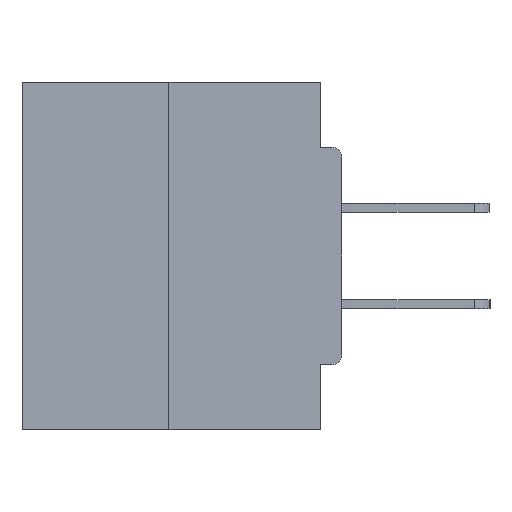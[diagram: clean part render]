
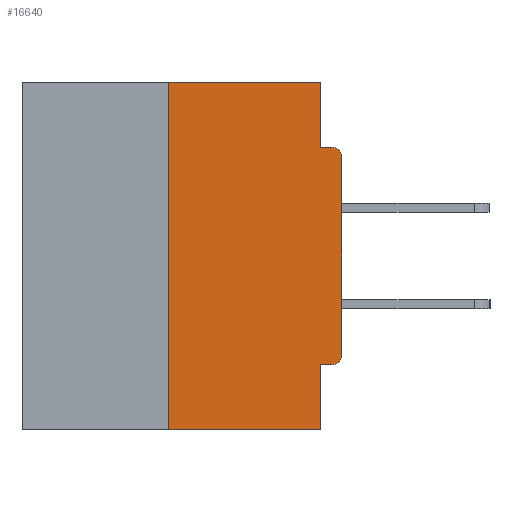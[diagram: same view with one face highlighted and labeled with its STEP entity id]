
A CAD part, left-side view. The second image highlights one B-rep face of the part: STEP entity #16640.
In plain terms, the highlighted planar face has unit normal (-1, 0, 0).
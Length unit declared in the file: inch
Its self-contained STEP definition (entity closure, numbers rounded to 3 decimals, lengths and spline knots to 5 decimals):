
#1625 = ORIENTED_EDGE ( 'NONE', *, *, #4944, .F. ) ;
#2277 = CIRCLE ( 'NONE', #15593, 0.015 ) ;
#2612 = VERTEX_POINT ( 'NONE', #27518 ) ;
#2887 = DIRECTION ( 'NONE',  ( -1., 0., 0. ) ) ;
#3757 = VERTEX_POINT ( 'NONE', #20801 ) ;
#3914 = DIRECTION ( 'NONE',  ( 0., -1., 0. ) ) ;
#4056 = CARTESIAN_POINT ( 'NONE',  ( 0., 0., -0.3915 ) ) ;
#4229 = VERTEX_POINT ( 'NONE', #33906 ) ;
#4318 = DIRECTION ( 'NONE',  ( 0., 0., -1. ) ) ;
#4486 = ORIENTED_EDGE ( 'NONE', *, *, #28692, .F. ) ;
#4723 = LINE ( 'NONE', #15482, #22766 ) ;
#4836 = CARTESIAN_POINT ( 'NONE',  ( 0., 0., -0.1085 ) ) ;
#4944 = EDGE_CURVE ( 'NONE', #12476, #11178, #12826, .T. ) ;
#5734 = ORIENTED_EDGE ( 'NONE', *, *, #23416, .F. ) ;
#6094 = VECTOR ( 'NONE', #3914, 39.37008 ) ;
#6627 = LINE ( 'NONE', #19983, #21672 ) ;
#7762 = DIRECTION ( 'NONE',  ( 1., 0., 0. ) ) ;
#8861 = VERTEX_POINT ( 'NONE', #4056 ) ;
#9237 = EDGE_CURVE ( 'NONE', #21258, #32486, #2277, .T. ) ;
#9597 = LINE ( 'NONE', #22953, #24629 ) ;
#9825 = VECTOR ( 'NONE', #4318, 39.37008 ) ;
#10478 = CIRCLE ( 'NONE', #27657, 0.015 ) ;
#10532 = CARTESIAN_POINT ( 'NONE',  ( 0., 0.031, 0. ) ) ;
#10607 = CARTESIAN_POINT ( 'NONE',  ( 0., 0., -0.4065 ) ) ;
#10702 = CARTESIAN_POINT ( 'NONE',  ( 0., 0.25, -0.5 ) ) ;
#11178 = VERTEX_POINT ( 'NONE', #13325 ) ;
#11704 = AXIS2_PLACEMENT_3D ( 'NONE', #15598, #7762, #18367 ) ;
#12137 = ORIENTED_EDGE ( 'NONE', *, *, #33587, .F. ) ;
#12476 = VERTEX_POINT ( 'NONE', #10702 ) ;
#12641 = PLANE ( 'NONE',  #11704 ) ;
#12826 = LINE ( 'NONE', #15449, #31124 ) ;
#12833 = CARTESIAN_POINT ( 'NONE',  ( 0., 0.46, 0. ) ) ;
#12966 = CARTESIAN_POINT ( 'NONE',  ( 0., 0.031, -0.5 ) ) ;
#13325 = CARTESIAN_POINT ( 'NONE',  ( 0., 0.25, 0. ) ) ;
#14563 = DIRECTION ( 'NONE',  ( 0., 0., -1. ) ) ;
#14739 = CARTESIAN_POINT ( 'NONE',  ( 0., 0.031, 0. ) ) ;
#15449 = CARTESIAN_POINT ( 'NONE',  ( 0., 0.25, 0. ) ) ;
#15482 = CARTESIAN_POINT ( 'NONE',  ( 0., 0., -0.0935 ) ) ;
#15593 = AXIS2_PLACEMENT_3D ( 'NONE', #16087, #2887, #26626 ) ;
#15598 = CARTESIAN_POINT ( 'NONE',  ( 0., 0.46, 0. ) ) ;
#16087 = CARTESIAN_POINT ( 'NONE',  ( 0., 0.015, -0.1085 ) ) ;
#16595 = VERTEX_POINT ( 'NONE', #10532 ) ;
#16640 = ADVANCED_FACE ( 'NONE', ( #21136 ), #12641, .F. ) ;
#17228 = DIRECTION ( 'NONE',  ( 0., 0., -1. ) ) ;
#18087 = DIRECTION ( 'NONE',  ( 0., -1., 0. ) ) ;
#18219 = LINE ( 'NONE', #12833, #22605 ) ;
#18367 = DIRECTION ( 'NONE',  ( 0., 0., -1. ) ) ;
#18599 = LINE ( 'NONE', #10607, #23831 ) ;
#19044 = ORIENTED_EDGE ( 'NONE', *, *, #32933, .T. ) ;
#19983 = CARTESIAN_POINT ( 'NONE',  ( 0., 0.031, -0.5 ) ) ;
#20801 = CARTESIAN_POINT ( 'NONE',  ( 0., 0.015, -0.4065 ) ) ;
#21136 = FACE_OUTER_BOUND ( 'NONE', #26148, .T. ) ;
#21223 = VERTEX_POINT ( 'NONE', #12966 ) ;
#21258 = VERTEX_POINT ( 'NONE', #4836 ) ;
#21667 = ORIENTED_EDGE ( 'NONE', *, *, #22463, .T. ) ;
#21672 = VECTOR ( 'NONE', #17228, 39.37008 ) ;
#21806 = LINE ( 'NONE', #27652, #6094 ) ;
#22463 = EDGE_CURVE ( 'NONE', #3757, #8861, #10478, .T. ) ;
#22605 = VECTOR ( 'NONE', #33959, 39.37008 ) ;
#22766 = VECTOR ( 'NONE', #18087, 39.37008 ) ;
#22953 = CARTESIAN_POINT ( 'NONE',  ( 0., 0., 0. ) ) ;
#23416 = EDGE_CURVE ( 'NONE', #2612, #32486, #4723, .T. ) ;
#23831 = VECTOR ( 'NONE', #31560, 39.37008 ) ;
#24629 = VECTOR ( 'NONE', #27610, 39.37008 ) ;
#25316 = EDGE_CURVE ( 'NONE', #4229, #21223, #6627, .T. ) ;
#25901 = ORIENTED_EDGE ( 'NONE', *, *, #25316, .F. ) ;
#26148 = EDGE_LOOP ( 'NONE', ( #4486, #1625, #19044, #25901, #12137, #21667, #29848, #29874, #5734, #27010 ) ) ;
#26626 = DIRECTION ( 'NONE',  ( 0., 0., -1. ) ) ;
#27010 = ORIENTED_EDGE ( 'NONE', *, *, #28874, .F. ) ;
#27518 = CARTESIAN_POINT ( 'NONE',  ( 0., 0.031, -0.0935 ) ) ;
#27523 = DIRECTION ( 'NONE',  ( -1., 0., 0. ) ) ;
#27539 = LINE ( 'NONE', #14739, #9825 ) ;
#27610 = DIRECTION ( 'NONE',  ( 0., 0., 1. ) ) ;
#27652 = CARTESIAN_POINT ( 'NONE',  ( 0., 0.46, -0.5 ) ) ;
#27657 = AXIS2_PLACEMENT_3D ( 'NONE', #33577, #27523, #14563 ) ;
#28692 = EDGE_CURVE ( 'NONE', #11178, #16595, #18219, .T. ) ;
#28874 = EDGE_CURVE ( 'NONE', #16595, #2612, #27539, .T. ) ;
#29848 = ORIENTED_EDGE ( 'NONE', *, *, #32140, .T. ) ;
#29874 = ORIENTED_EDGE ( 'NONE', *, *, #9237, .T. ) ;
#29963 = CARTESIAN_POINT ( 'NONE',  ( 0., 0.015, -0.0935 ) ) ;
#31124 = VECTOR ( 'NONE', #31343, 39.37008 ) ;
#31343 = DIRECTION ( 'NONE',  ( 0., 0., 1. ) ) ;
#31560 = DIRECTION ( 'NONE',  ( 0., 1., 0. ) ) ;
#32140 = EDGE_CURVE ( 'NONE', #8861, #21258, #9597, .T. ) ;
#32486 = VERTEX_POINT ( 'NONE', #29963 ) ;
#32933 = EDGE_CURVE ( 'NONE', #12476, #21223, #21806, .T. ) ;
#33577 = CARTESIAN_POINT ( 'NONE',  ( 0., 0.015, -0.3915 ) ) ;
#33587 = EDGE_CURVE ( 'NONE', #3757, #4229, #18599, .T. ) ;
#33906 = CARTESIAN_POINT ( 'NONE',  ( 0., 0.031, -0.4065 ) ) ;
#33959 = DIRECTION ( 'NONE',  ( 0., -1., 0. ) ) ;
